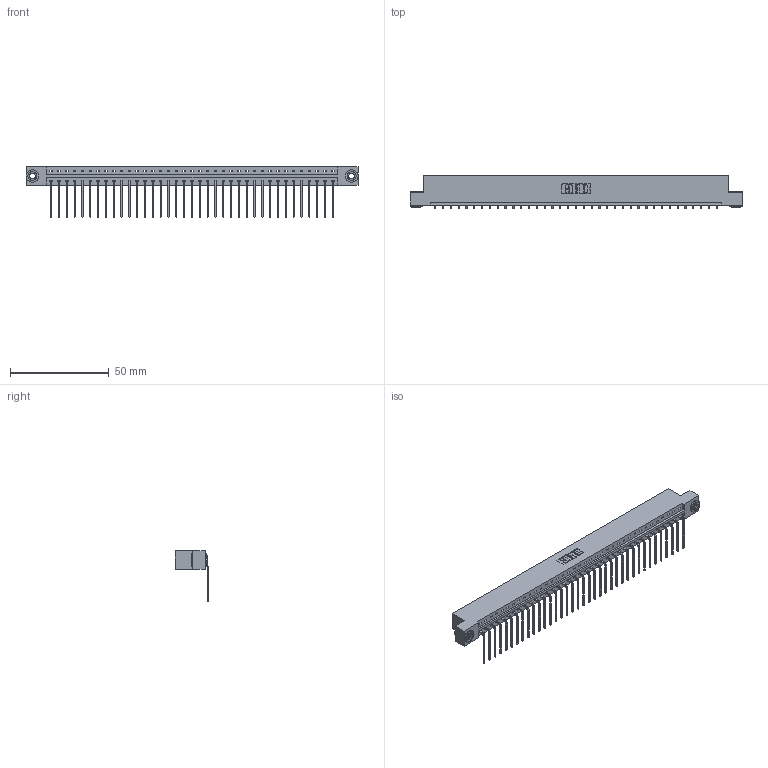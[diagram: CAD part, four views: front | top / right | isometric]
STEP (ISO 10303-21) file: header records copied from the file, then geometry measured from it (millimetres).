
FILE_DESCRIPTION (( 'STEP AP203' ), '1' );
FILE_NAME ('833-037-559-103.STEP', '2020-06-03T05:52:29', ( '' ), ( '' ), 'SwSTEP 2.0', 'SolidWorks 2020', '' );
FILE_SCHEMA (( 'CONFIG_CONTROL_DESIGN' ));
Length unit declared in the file: inch
Products named in the file (4): 833-037-559-103; 833 Part_Flush - .156 Dia - TH; 345-250-002_345-250-002-102; 345-292-001_558 559 Tail - 1
Assembly tree (40 placements, depth 2):
  833-037-559-103
    833 Part_Flush - .156 Dia - TH
    345-292-001_558 559 Tail - 1  x37
    345-250-002_345-250-002-102  x2
Bounding box: 168.15 x 17.09 x 25.53 mm (x, y, z)
Volume: 17020.1 mm3; surface area: 19366.3 mm2
Topology: 40 solids, 40 shells, 2372 faces, 7121 edges, 4694 vertices
Faces by surface type: plane 1708, cylinder 656, cone 8
Entity records: 24000 total; most frequent: CARTESIAN_POINT 4120, ORIENTED_EDGE 4086, DIRECTION 3519, EDGE_CURVE 2043, LINE 1891, VECTOR 1891, VERTEX_POINT 1358, AXIS2_PLACEMENT_3D 814
